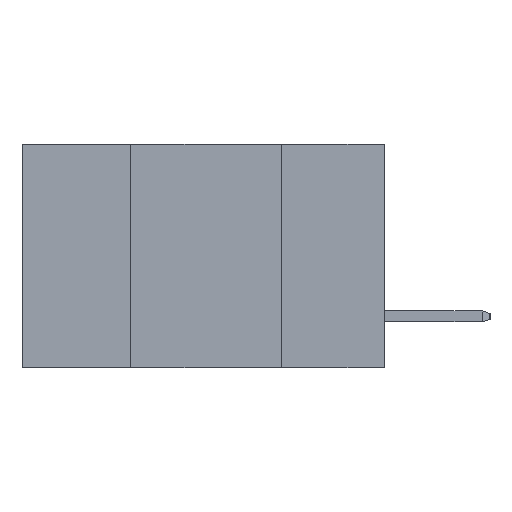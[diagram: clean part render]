
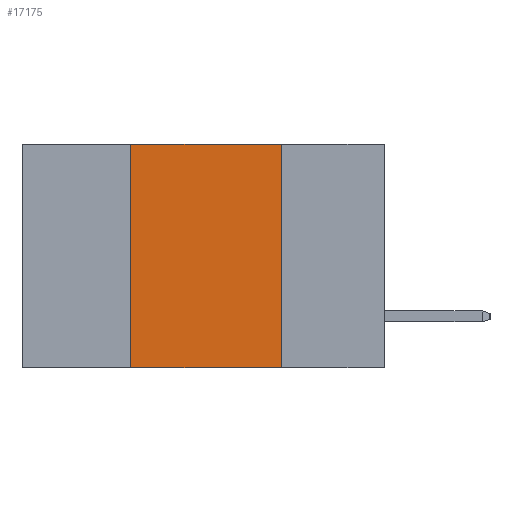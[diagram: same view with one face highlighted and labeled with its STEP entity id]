
A CAD part, left-side view. The second image highlights one B-rep face of the part: STEP entity #17175.
In plain terms, the highlighted planar face has unit normal (-1, 0, 0).
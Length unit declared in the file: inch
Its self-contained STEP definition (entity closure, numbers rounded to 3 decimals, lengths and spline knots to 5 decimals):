
#1192 = VECTOR ( 'NONE', #18759, 39.37008 ) ;
#1326 = FACE_OUTER_BOUND ( 'NONE', #12246, .T. ) ;
#1475 = EDGE_CURVE ( 'NONE', #17373, #13762, #6988, .T. ) ;
#1698 = CARTESIAN_POINT ( 'NONE',  ( 0., 0.17, -0.37 ) ) ;
#2502 = CARTESIAN_POINT ( 'NONE',  ( 0., 0.17, 0. ) ) ;
#3894 = CARTESIAN_POINT ( 'NONE',  ( 0., 0.42, -0.37 ) ) ;
#3964 = PLANE ( 'NONE',  #12972 ) ;
#5798 = CARTESIAN_POINT ( 'NONE',  ( 0., 0.6, 0. ) ) ;
#6087 = CARTESIAN_POINT ( 'NONE',  ( 0., 0.42, -0.37 ) ) ;
#6444 = EDGE_CURVE ( 'NONE', #17143, #7683, #13710, .T. ) ;
#6944 = CARTESIAN_POINT ( 'NONE',  ( 0., 0.17, -0.37 ) ) ;
#6988 = LINE ( 'NONE', #5798, #16038 ) ;
#7054 = DIRECTION ( 'NONE',  ( 0., -1., 0. ) ) ;
#7199 = CARTESIAN_POINT ( 'NONE',  ( 0., 0.6, -0.37 ) ) ;
#7440 = CARTESIAN_POINT ( 'NONE',  ( 0., 0.6, 0. ) ) ;
#7683 = VERTEX_POINT ( 'NONE', #1698 ) ;
#7718 = ORIENTED_EDGE ( 'NONE', *, *, #14478, .F. ) ;
#8669 = VECTOR ( 'NONE', #20624, 39.37008 ) ;
#8706 = LINE ( 'NONE', #6944, #1192 ) ;
#9215 = DIRECTION ( 'NONE',  ( 0., 0., -1. ) ) ;
#11776 = CARTESIAN_POINT ( 'NONE',  ( 0., 0.42, 0. ) ) ;
#12246 = EDGE_LOOP ( 'NONE', ( #21150, #19300, #7718, #14507 ) ) ;
#12972 = AXIS2_PLACEMENT_3D ( 'NONE', #7440, #19192, #9215 ) ;
#13710 = LINE ( 'NONE', #7199, #8669 ) ;
#13762 = VERTEX_POINT ( 'NONE', #2502 ) ;
#14478 = EDGE_CURVE ( 'NONE', #17143, #17373, #16299, .T. ) ;
#14507 = ORIENTED_EDGE ( 'NONE', *, *, #6444, .T. ) ;
#16038 = VECTOR ( 'NONE', #7054, 39.37008 ) ;
#16299 = LINE ( 'NONE', #6087, #20145 ) ;
#17143 = VERTEX_POINT ( 'NONE', #3894 ) ;
#17175 = ADVANCED_FACE ( 'NONE', ( #1326 ), #3964, .F. ) ;
#17373 = VERTEX_POINT ( 'NONE', #11776 ) ;
#18759 = DIRECTION ( 'NONE',  ( 0., 0., -1. ) ) ;
#18902 = EDGE_CURVE ( 'NONE', #13762, #7683, #8706, .T. ) ;
#19192 = DIRECTION ( 'NONE',  ( 1., 0., 0. ) ) ;
#19300 = ORIENTED_EDGE ( 'NONE', *, *, #1475, .F. ) ;
#19572 = DIRECTION ( 'NONE',  ( 0., 0., 1. ) ) ;
#20145 = VECTOR ( 'NONE', #19572, 39.37008 ) ;
#20624 = DIRECTION ( 'NONE',  ( 0., -1., 0. ) ) ;
#21150 = ORIENTED_EDGE ( 'NONE', *, *, #18902, .F. ) ;
